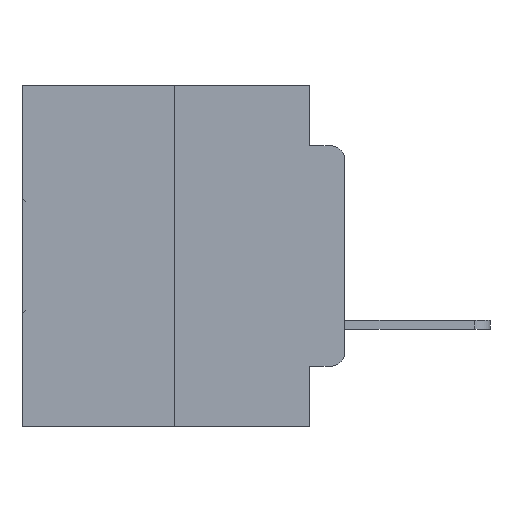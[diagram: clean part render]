
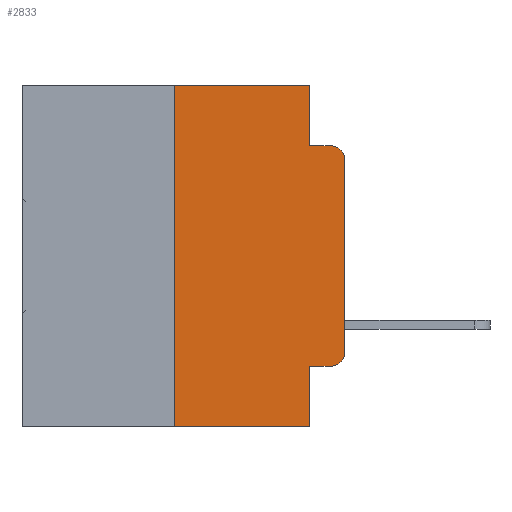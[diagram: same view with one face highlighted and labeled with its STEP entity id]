
A CAD part, left-side view. The second image highlights one B-rep face of the part: STEP entity #2833.
In plain terms, the highlighted planar face has unit normal (-1, 0, 0).
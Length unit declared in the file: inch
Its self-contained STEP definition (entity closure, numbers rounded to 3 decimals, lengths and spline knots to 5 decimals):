
#28 = DIRECTION ( 'NONE',  ( 1., 0., 0. ) ) ;
#202 = VECTOR ( 'NONE', #23550, 39.37008 ) ;
#549 = CARTESIAN_POINT ( 'NONE',  ( 0., 0.051, 0. ) ) ;
#681 = VECTOR ( 'NONE', #14771, 39.37008 ) ;
#1740 = DIRECTION ( 'NONE',  ( 0., 0., -1. ) ) ;
#1934 = EDGE_CURVE ( 'NONE', #17223, #12133, #30128, .T. ) ;
#1941 = VERTEX_POINT ( 'NONE', #10162 ) ;
#2833 = ADVANCED_FACE ( 'NONE', ( #30068 ), #32655, .F. ) ;
#2863 = ORIENTED_EDGE ( 'NONE', *, *, #19154, .F. ) ;
#3284 = VERTEX_POINT ( 'NONE', #25974 ) ;
#3790 = VERTEX_POINT ( 'NONE', #14513 ) ;
#4146 = ORIENTED_EDGE ( 'NONE', *, *, #24335, .T. ) ;
#4419 = VECTOR ( 'NONE', #21139, 39.37008 ) ;
#5390 = CARTESIAN_POINT ( 'NONE',  ( 0., 0.473, -0.5 ) ) ;
#5746 = ORIENTED_EDGE ( 'NONE', *, *, #17124, .F. ) ;
#6763 = DIRECTION ( 'NONE',  ( 0., -1., 0. ) ) ;
#7450 = ORIENTED_EDGE ( 'NONE', *, *, #17611, .F. ) ;
#7511 = CARTESIAN_POINT ( 'NONE',  ( 0., 0.02, -0.0885 ) ) ;
#7651 = CARTESIAN_POINT ( 'NONE',  ( 0., 0.25, 0. ) ) ;
#8984 = CARTESIAN_POINT ( 'NONE',  ( 0., 0.02, -0.4115 ) ) ;
#9360 = CARTESIAN_POINT ( 'NONE',  ( 0., 0., -0.1085 ) ) ;
#9511 = ORIENTED_EDGE ( 'NONE', *, *, #18926, .F. ) ;
#9528 = CIRCLE ( 'NONE', #18676, 0.02 ) ;
#9530 = CARTESIAN_POINT ( 'NONE',  ( 0., 0.02, -0.3915 ) ) ;
#9835 = DIRECTION ( 'NONE',  ( 0., 0., -1. ) ) ;
#10059 = EDGE_CURVE ( 'NONE', #16724, #30396, #31086, .T. ) ;
#10064 = DIRECTION ( 'NONE',  ( -1., 0., 0. ) ) ;
#10162 = CARTESIAN_POINT ( 'NONE',  ( 0., 0.051, -0.4115 ) ) ;
#10842 = ORIENTED_EDGE ( 'NONE', *, *, #15865, .T. ) ;
#10975 = CARTESIAN_POINT ( 'NONE',  ( 0., 0., -0.3915 ) ) ;
#11093 = VECTOR ( 'NONE', #6763, 39.37008 ) ;
#11505 = VECTOR ( 'NONE', #25885, 39.37008 ) ;
#11665 = VECTOR ( 'NONE', #13823, 39.37008 ) ;
#12133 = VERTEX_POINT ( 'NONE', #10975 ) ;
#12207 = CARTESIAN_POINT ( 'NONE',  ( 0., 0., 0. ) ) ;
#13823 = DIRECTION ( 'NONE',  ( 0., 0., -1. ) ) ;
#13953 = VERTEX_POINT ( 'NONE', #27624 ) ;
#14513 = CARTESIAN_POINT ( 'NONE',  ( 0., 0.051, -0.5 ) ) ;
#14589 = DIRECTION ( 'NONE',  ( 0., 0., -1. ) ) ;
#14771 = DIRECTION ( 'NONE',  ( 0., 0., 1. ) ) ;
#15150 = AXIS2_PLACEMENT_3D ( 'NONE', #31938, #28, #14589 ) ;
#15560 = DIRECTION ( 'NONE',  ( 0., 0., -1. ) ) ;
#15865 = EDGE_CURVE ( 'NONE', #1941, #17223, #25881, .T. ) ;
#16724 = VERTEX_POINT ( 'NONE', #19411 ) ;
#17124 = EDGE_CURVE ( 'NONE', #3284, #13953, #31231, .T. ) ;
#17148 = LINE ( 'NONE', #5390, #22916 ) ;
#17223 = VERTEX_POINT ( 'NONE', #8984 ) ;
#17413 = EDGE_CURVE ( 'NONE', #27041, #21351, #9528, .T. ) ;
#17459 = DIRECTION ( 'NONE',  ( -1., 0., 0. ) ) ;
#17611 = EDGE_CURVE ( 'NONE', #1941, #3790, #24091, .T. ) ;
#17991 = EDGE_CURVE ( 'NONE', #12133, #27041, #20631, .T. ) ;
#18275 = LINE ( 'NONE', #25994, #4419 ) ;
#18676 = AXIS2_PLACEMENT_3D ( 'NONE', #31948, #17459, #1740 ) ;
#18740 = CARTESIAN_POINT ( 'NONE',  ( 0., 0.051, -0.4115 ) ) ;
#18926 = EDGE_CURVE ( 'NONE', #13953, #21351, #18275, .T. ) ;
#19154 = EDGE_CURVE ( 'NONE', #30396, #3284, #30722, .T. ) ;
#19411 = CARTESIAN_POINT ( 'NONE',  ( 0., 0.25, -0.5 ) ) ;
#19628 = CARTESIAN_POINT ( 'NONE',  ( 0., 0.473, 0. ) ) ;
#19853 = ORIENTED_EDGE ( 'NONE', *, *, #17991, .T. ) ;
#20558 = CARTESIAN_POINT ( 'NONE',  ( 0., 0.051, 0. ) ) ;
#20631 = LINE ( 'NONE', #12207, #681 ) ;
#20821 = DIRECTION ( 'NONE',  ( 0., -1., 0. ) ) ;
#21041 = CARTESIAN_POINT ( 'NONE',  ( 0., 0.25, 0. ) ) ;
#21139 = DIRECTION ( 'NONE',  ( 0., -1., 0. ) ) ;
#21351 = VERTEX_POINT ( 'NONE', #7511 ) ;
#22916 = VECTOR ( 'NONE', #20821, 39.37008 ) ;
#22967 = EDGE_LOOP ( 'NONE', ( #19853, #24080, #9511, #5746, #2863, #31979, #4146, #7450, #10842, #26380 ) ) ;
#23550 = DIRECTION ( 'NONE',  ( 0., -1., 0. ) ) ;
#24080 = ORIENTED_EDGE ( 'NONE', *, *, #17413, .T. ) ;
#24091 = LINE ( 'NONE', #20558, #29689 ) ;
#24335 = EDGE_CURVE ( 'NONE', #16724, #3790, #17148, .T. ) ;
#25826 = AXIS2_PLACEMENT_3D ( 'NONE', #9530, #10064, #9835 ) ;
#25881 = LINE ( 'NONE', #18740, #202 ) ;
#25885 = DIRECTION ( 'NONE',  ( 0., 0., 1. ) ) ;
#25974 = CARTESIAN_POINT ( 'NONE',  ( 0., 0.051, 0. ) ) ;
#25994 = CARTESIAN_POINT ( 'NONE',  ( 0., 0.051, -0.0885 ) ) ;
#26380 = ORIENTED_EDGE ( 'NONE', *, *, #1934, .T. ) ;
#27041 = VERTEX_POINT ( 'NONE', #9360 ) ;
#27624 = CARTESIAN_POINT ( 'NONE',  ( 0., 0.051, -0.0885 ) ) ;
#29689 = VECTOR ( 'NONE', #15560, 39.37008 ) ;
#30068 = FACE_OUTER_BOUND ( 'NONE', #22967, .T. ) ;
#30128 = CIRCLE ( 'NONE', #25826, 0.02 ) ;
#30396 = VERTEX_POINT ( 'NONE', #7651 ) ;
#30722 = LINE ( 'NONE', #19628, #11093 ) ;
#31086 = LINE ( 'NONE', #21041, #11505 ) ;
#31231 = LINE ( 'NONE', #549, #11665 ) ;
#31938 = CARTESIAN_POINT ( 'NONE',  ( 0., 0.473, 0. ) ) ;
#31948 = CARTESIAN_POINT ( 'NONE',  ( 0., 0.02, -0.1085 ) ) ;
#31979 = ORIENTED_EDGE ( 'NONE', *, *, #10059, .F. ) ;
#32655 = PLANE ( 'NONE',  #15150 ) ;
